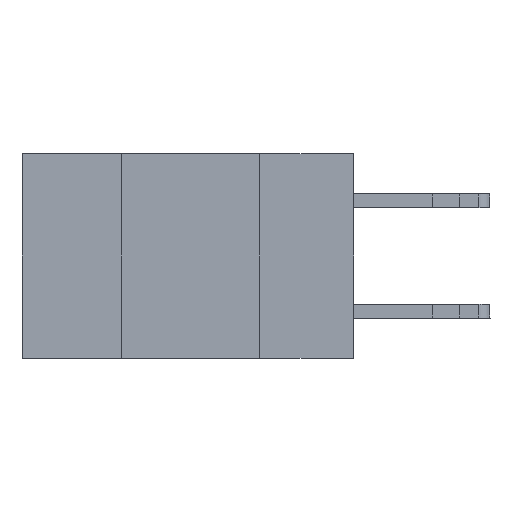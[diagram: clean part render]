
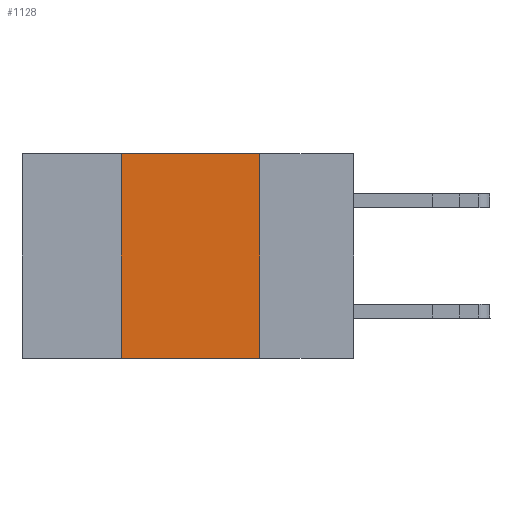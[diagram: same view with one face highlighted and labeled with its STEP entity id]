
A CAD part, left-side view. The second image highlights one B-rep face of the part: STEP entity #1128.
In plain terms, the highlighted planar face has unit normal (-1, 0, 0).
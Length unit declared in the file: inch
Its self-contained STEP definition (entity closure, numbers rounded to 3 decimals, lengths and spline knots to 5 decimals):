
#1128 = ADVANCED_FACE ( 'NONE', ( #8304 ), #1754, .F. ) ;
#1166 = DIRECTION ( 'NONE',  ( 0., 0., 1. ) ) ;
#1754 = PLANE ( 'NONE',  #12810 ) ;
#1792 = DIRECTION ( 'NONE',  ( 0., -1., 0. ) ) ;
#2422 = VERTEX_POINT ( 'NONE', #14550 ) ;
#3320 = VERTEX_POINT ( 'NONE', #10834 ) ;
#4015 = CARTESIAN_POINT ( 'NONE',  ( 0., 0.42, 0. ) ) ;
#4901 = LINE ( 'NONE', #13853, #11251 ) ;
#5232 = ORIENTED_EDGE ( 'NONE', *, *, #14043, .F. ) ;
#5365 = CARTESIAN_POINT ( 'NONE',  ( 0., 0.6, -0.37 ) ) ;
#5849 = EDGE_CURVE ( 'NONE', #2422, #3320, #16513, .T. ) ;
#6185 = LINE ( 'NONE', #16617, #9215 ) ;
#7222 = ORIENTED_EDGE ( 'NONE', *, *, #11776, .F. ) ;
#8304 = FACE_OUTER_BOUND ( 'NONE', #15365, .T. ) ;
#8885 = CARTESIAN_POINT ( 'NONE',  ( 0., 0.6, 0. ) ) ;
#9215 = VECTOR ( 'NONE', #1166, 39.37008 ) ;
#9367 = EDGE_CURVE ( 'NONE', #13495, #11871, #10306, .T. ) ;
#9650 = VECTOR ( 'NONE', #1792, 39.37008 ) ;
#10306 = LINE ( 'NONE', #8885, #13644 ) ;
#10764 = DIRECTION ( 'NONE',  ( 0., 0., -1. ) ) ;
#10834 = CARTESIAN_POINT ( 'NONE',  ( 0., 0.17, -0.37 ) ) ;
#11251 = VECTOR ( 'NONE', #15184, 39.37008 ) ;
#11776 = EDGE_CURVE ( 'NONE', #11871, #3320, #4901, .T. ) ;
#11871 = VERTEX_POINT ( 'NONE', #12746 ) ;
#11911 = CARTESIAN_POINT ( 'NONE',  ( 0., 0.6, 0. ) ) ;
#12746 = CARTESIAN_POINT ( 'NONE',  ( 0., 0.17, 0. ) ) ;
#12810 = AXIS2_PLACEMENT_3D ( 'NONE', #11911, #16370, #10764 ) ;
#13272 = ORIENTED_EDGE ( 'NONE', *, *, #5849, .T. ) ;
#13495 = VERTEX_POINT ( 'NONE', #4015 ) ;
#13644 = VECTOR ( 'NONE', #16587, 39.37008 ) ;
#13853 = CARTESIAN_POINT ( 'NONE',  ( 0., 0.17, 0. ) ) ;
#14043 = EDGE_CURVE ( 'NONE', #2422, #13495, #6185, .T. ) ;
#14291 = ORIENTED_EDGE ( 'NONE', *, *, #9367, .F. ) ;
#14550 = CARTESIAN_POINT ( 'NONE',  ( 0., 0.42, -0.37 ) ) ;
#15184 = DIRECTION ( 'NONE',  ( 0., 0., -1. ) ) ;
#15365 = EDGE_LOOP ( 'NONE', ( #7222, #14291, #5232, #13272 ) ) ;
#16370 = DIRECTION ( 'NONE',  ( 1., 0., 0. ) ) ;
#16513 = LINE ( 'NONE', #5365, #9650 ) ;
#16587 = DIRECTION ( 'NONE',  ( 0., -1., 0. ) ) ;
#16617 = CARTESIAN_POINT ( 'NONE',  ( 0., 0.42, 0. ) ) ;
